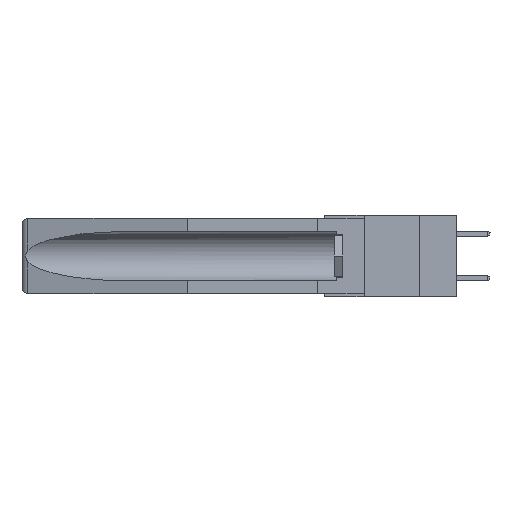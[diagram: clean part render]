
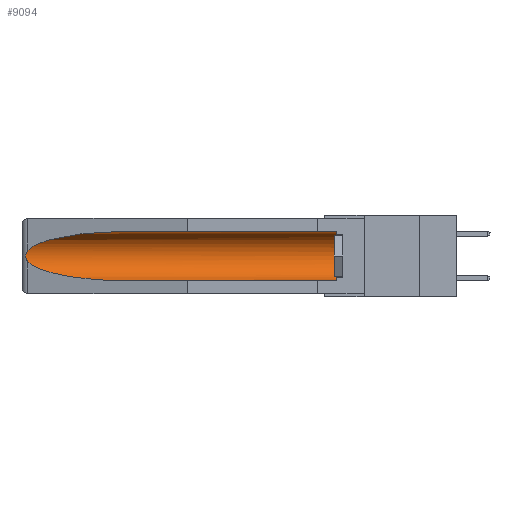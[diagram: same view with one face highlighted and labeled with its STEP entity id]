
A CAD part, left-side view. The second image highlights one B-rep face of the part: STEP entity #9094.
In plain terms, the highlighted cylindrical face has radius 2.857 mm (diameter 5.715 mm), a partial arc.
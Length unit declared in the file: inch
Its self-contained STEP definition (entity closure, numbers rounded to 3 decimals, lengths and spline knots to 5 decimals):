
#906 = CARTESIAN_POINT ( 'NONE',  ( 0.26597, 1.52961, -0.15275 ) ) ;
#1110 = CARTESIAN_POINT ( 'NONE',  ( 0.155, 1.07973, -0.284 ) ) ;
#1473 = CARTESIAN_POINT ( 'NONE',  ( 0.26537, 1.52718, -0.19328 ) ) ;
#1653 = EDGE_CURVE ( 'NONE', #25886, #9625, #3693, .T. ) ;
#1928 = CIRCLE ( 'NONE', #20445, 0.1125 ) ;
#2240 = ORIENTED_EDGE ( 'NONE', *, *, #7671, .T. ) ;
#2347 = CARTESIAN_POINT ( 'NONE',  ( 0.155, 0.126, -0.284 ) ) ;
#3693 = LINE ( 'NONE', #16244, #15156 ) ;
#4053 = ORIENTED_EDGE ( 'NONE', *, *, #21667, .T. ) ;
#4079 = CARTESIAN_POINT ( 'NONE',  ( 0.21114, 1.30732, -0.284 ) ) ;
#4431 = CARTESIAN_POINT ( 'NONE',  ( 0.155, 1.07973, -0.284 ) ) ;
#4739 = EDGE_LOOP ( 'NONE', ( #25676, #28639, #2240, #7513, #4053, #29675 ) ) ;
#6314 = CARTESIAN_POINT ( 'NONE',  ( 0.2675, 1.53308, -0.17534 ) ) ;
#6848 = FACE_OUTER_BOUND ( 'NONE', #4739, .T. ) ;
#7513 = ORIENTED_EDGE ( 'NONE', *, *, #1653, .F. ) ;
#7671 = EDGE_CURVE ( 'NONE', #32101, #9625, #26724, .T. ) ;
#8146 =( BOUNDED_CURVE ( )  B_SPLINE_CURVE ( 3, ( #28399, #12636, #8888, #20525 ),
 .UNSPECIFIED., .F., .F. ) 
 B_SPLINE_CURVE_WITH_KNOTS ( ( 4, 4 ),
 ( 4.71239, 6.08839 ),
 .UNSPECIFIED. ) 
 CURVE ( )  GEOMETRIC_REPRESENTATION_ITEM ( )  RATIONAL_B_SPLINE_CURVE ( ( 1., 0.848, 0.848, 1. ) ) 
 REPRESENTATION_ITEM ( '' )  );
#8169 = VERTEX_POINT ( 'NONE', #18233 ) ;
#8888 = CARTESIAN_POINT ( 'NONE',  ( 0.25451, 1.48313, -0.09465 ) ) ;
#8920 = CARTESIAN_POINT ( 'NONE',  ( 0.26537, 1.52718, -0.14972 ) ) ;
#9094 = ADVANCED_FACE ( 'NONE', ( #6848 ), #31453, .F. ) ;
#9625 = VERTEX_POINT ( 'NONE', #4431 ) ;
#11112 = DIRECTION ( 'NONE',  ( 0., 1., 0. ) ) ;
#11492 = LINE ( 'NONE', #18800, #32373 ) ;
#12091 = CARTESIAN_POINT ( 'NONE',  ( 0.25451, 1.48313, -0.24835 ) ) ;
#12636 = CARTESIAN_POINT ( 'NONE',  ( 0.21114, 1.30732, -0.059 ) ) ;
#13664 = DIRECTION ( 'NONE',  ( 0., -1., 0. ) ) ;
#15156 = VECTOR ( 'NONE', #11112, 39.37008 ) ;
#15617 = VERTEX_POINT ( 'NONE', #23982 ) ;
#16244 = CARTESIAN_POINT ( 'NONE',  ( 0.155, -0.30754, -0.284 ) ) ;
#16285 = DIRECTION ( 'NONE',  ( 0., 0., 1. ) ) ;
#17370 = B_SPLINE_CURVE_WITH_KNOTS ( 'NONE', 3,
 ( #8920, #906, #19374, #22174, #19484, #6314, #22061, #20049, #33307, #1473 ),
 .UNSPECIFIED., .F., .F.,
 ( 4, 2, 2, 2, 4 ),
 ( 0., 0.00029, 0.00058, 0.00087, 0.00117 ),
 .UNSPECIFIED. ) ;
#17636 = DIRECTION ( 'NONE',  ( 0., 0., 1. ) ) ;
#18233 = CARTESIAN_POINT ( 'NONE',  ( 0.155, 1.07973, -0.059 ) ) ;
#18800 = CARTESIAN_POINT ( 'NONE',  ( 0.155, -0.30754, -0.059 ) ) ;
#19374 = CARTESIAN_POINT ( 'NONE',  ( 0.26654, 1.53092, -0.15636 ) ) ;
#19484 = CARTESIAN_POINT ( 'NONE',  ( 0.2675, 1.53308, -0.16763 ) ) ;
#20049 = CARTESIAN_POINT ( 'NONE',  ( 0.26655, 1.53094, -0.18657 ) ) ;
#20445 = AXIS2_PLACEMENT_3D ( 'NONE', #29406, #13664, #16285 ) ;
#20525 = CARTESIAN_POINT ( 'NONE',  ( 0.26537, 1.52718, -0.14972 ) ) ;
#20812 = CARTESIAN_POINT ( 'NONE',  ( 0.155, 0.126, -0.059 ) ) ;
#21667 = EDGE_CURVE ( 'NONE', #25886, #30414, #1928, .T. ) ;
#22061 = CARTESIAN_POINT ( 'NONE',  ( 0.2673, 1.53269, -0.17917 ) ) ;
#22174 = CARTESIAN_POINT ( 'NONE',  ( 0.2673, 1.5327, -0.16383 ) ) ;
#22459 = EDGE_CURVE ( 'NONE', #8169, #15617, #8146, .T. ) ;
#23982 = CARTESIAN_POINT ( 'NONE',  ( 0.26537, 1.52718, -0.14972 ) ) ;
#24434 = CARTESIAN_POINT ( 'NONE',  ( 0.26537, 1.52718, -0.19328 ) ) ;
#25676 = ORIENTED_EDGE ( 'NONE', *, *, #22459, .T. ) ;
#25886 = VERTEX_POINT ( 'NONE', #2347 ) ;
#26724 =( BOUNDED_CURVE ( )  B_SPLINE_CURVE ( 3, ( #24434, #12091, #4079, #1110 ),
 .UNSPECIFIED., .F., .F. ) 
 B_SPLINE_CURVE_WITH_KNOTS ( ( 4, 4 ),
 ( 0.1948, 1.5708 ),
 .UNSPECIFIED. ) 
 CURVE ( )  GEOMETRIC_REPRESENTATION_ITEM ( )  RATIONAL_B_SPLINE_CURVE ( ( 1., 0.848, 0.848, 1. ) ) 
 REPRESENTATION_ITEM ( '' )  );
#26866 = EDGE_CURVE ( 'NONE', #15617, #32101, #17370, .T. ) ;
#28285 = AXIS2_PLACEMENT_3D ( 'NONE', #30959, #33013, #17636 ) ;
#28399 = CARTESIAN_POINT ( 'NONE',  ( 0.155, 1.07973, -0.059 ) ) ;
#28639 = ORIENTED_EDGE ( 'NONE', *, *, #26866, .T. ) ;
#29406 = CARTESIAN_POINT ( 'NONE',  ( 0.155, 0.126, -0.1715 ) ) ;
#29675 = ORIENTED_EDGE ( 'NONE', *, *, #30982, .T. ) ;
#30414 = VERTEX_POINT ( 'NONE', #20812 ) ;
#30959 = CARTESIAN_POINT ( 'NONE',  ( 0.155, -0.30754, -0.1715 ) ) ;
#30982 = EDGE_CURVE ( 'NONE', #30414, #8169, #11492, .T. ) ;
#31453 = CYLINDRICAL_SURFACE ( 'NONE', #28285, 0.1125 ) ;
#31866 = CARTESIAN_POINT ( 'NONE',  ( 0.26537, 1.52718, -0.19328 ) ) ;
#32101 = VERTEX_POINT ( 'NONE', #31866 ) ;
#32373 = VECTOR ( 'NONE', #32429, 39.37008 ) ;
#32429 = DIRECTION ( 'NONE',  ( 0., 1., 0. ) ) ;
#33013 = DIRECTION ( 'NONE',  ( 0., 1., 0. ) ) ;
#33307 = CARTESIAN_POINT ( 'NONE',  ( 0.26597, 1.5296, -0.19026 ) ) ;
